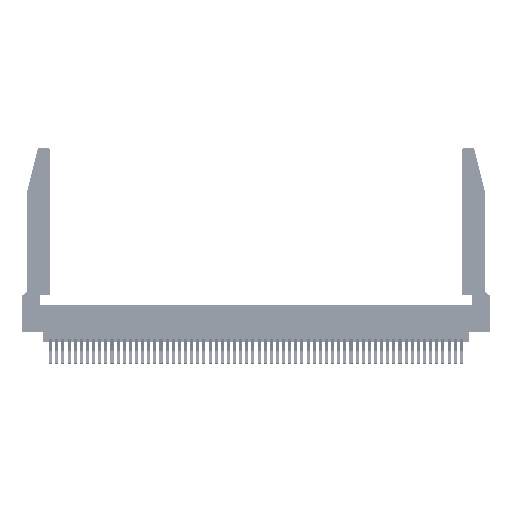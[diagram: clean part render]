
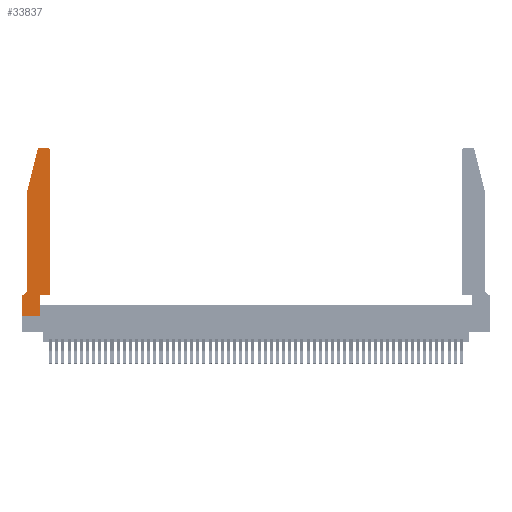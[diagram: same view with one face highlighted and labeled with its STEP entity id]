
A CAD part, top view. The second image highlights one B-rep face of the part: STEP entity #33837.
In plain terms, the highlighted planar face has unit normal (0, 0, 1).
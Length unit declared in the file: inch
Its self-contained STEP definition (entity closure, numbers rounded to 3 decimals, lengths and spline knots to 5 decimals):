
#17 = CARTESIAN_POINT ( 'NONE',  ( 0.2865, 0., 0.37 ) ) ;
#1931 = LINE ( 'NONE', #52127, #19778 ) ;
#2562 = VERTEX_POINT ( 'NONE', #24021 ) ;
#3129 = CARTESIAN_POINT ( 'NONE',  ( 0.4205, 2.75, 0.37 ) ) ;
#3317 = EDGE_CURVE ( 'NONE', #7591, #2562, #39348, .T. ) ;
#3468 = CARTESIAN_POINT ( 'NONE',  ( 0.4205, 2.72, 0.37 ) ) ;
#4200 = ORIENTED_EDGE ( 'NONE', *, *, #9746, .T. ) ;
#6083 = DIRECTION ( 'NONE',  ( 0., 1., 0. ) ) ;
#6955 = CARTESIAN_POINT ( 'NONE',  ( 0.2865, 0.35, 0.37 ) ) ;
#7202 = CIRCLE ( 'NONE', #25815, 0.03 ) ;
#7223 = AXIS2_PLACEMENT_3D ( 'NONE', #47999, #27829, #48746 ) ;
#7579 = EDGE_CURVE ( 'NONE', #15162, #51582, #19291, .T. ) ;
#7591 = VERTEX_POINT ( 'NONE', #15389 ) ;
#7745 = DIRECTION ( 'NONE',  ( 0., 0., 1. ) ) ;
#7972 = EDGE_CURVE ( 'NONE', #21771, #21928, #25898, .T. ) ;
#9334 = DIRECTION ( 'NONE',  ( -1., 0., 0. ) ) ;
#9746 = EDGE_CURVE ( 'NONE', #21928, #7591, #7202, .T. ) ;
#13194 = EDGE_CURVE ( 'NONE', #38398, #21771, #14257, .T. ) ;
#13204 = EDGE_CURVE ( 'NONE', #25595, #15162, #15594, .T. ) ;
#13573 = VERTEX_POINT ( 'NONE', #6955 ) ;
#14257 = CIRCLE ( 'NONE', #15981, 0.03 ) ;
#14456 = VERTEX_POINT ( 'NONE', #46178 ) ;
#15027 = CARTESIAN_POINT ( 'NONE',  ( 0., 0., 0.37 ) ) ;
#15162 = VERTEX_POINT ( 'NONE', #33357 ) ;
#15389 = CARTESIAN_POINT ( 'NONE',  ( 0.25487, 2.72718, 0.37 ) ) ;
#15594 = LINE ( 'NONE', #50302, #30167 ) ;
#15723 = ORIENTED_EDGE ( 'NONE', *, *, #7579, .T. ) ;
#15868 = ORIENTED_EDGE ( 'NONE', *, *, #22685, .T. ) ;
#15981 = AXIS2_PLACEMENT_3D ( 'NONE', #3468, #7745, #45841 ) ;
#16639 = EDGE_CURVE ( 'NONE', #51582, #37300, #1931, .T. ) ;
#17595 = EDGE_LOOP ( 'NONE', ( #52752, #4200, #49155, #15868, #50576, #19796, #15723, #22686, #35357, #24767, #21542, #46918 ) ) ;
#17770 = CARTESIAN_POINT ( 'NONE',  ( 0., 0., 0.37 ) ) ;
#18060 = LINE ( 'NONE', #51191, #53843 ) ;
#18257 = DIRECTION ( 'NONE',  ( -1., 0., 0. ) ) ;
#18615 = CARTESIAN_POINT ( 'NONE',  ( 0.0055, 0.42, 0.37 ) ) ;
#19123 = DIRECTION ( 'NONE',  ( 1., 0., 0. ) ) ;
#19291 = LINE ( 'NONE', #15027, #24624 ) ;
#19778 = VECTOR ( 'NONE', #19123, 39.37008 ) ;
#19796 = ORIENTED_EDGE ( 'NONE', *, *, #13204, .T. ) ;
#19903 = LINE ( 'NONE', #42523, #31259 ) ;
#20831 = VECTOR ( 'NONE', #24140, 39.37008 ) ;
#21542 = ORIENTED_EDGE ( 'NONE', *, *, #47731, .T. ) ;
#21729 = CARTESIAN_POINT ( 'NONE',  ( 0.2605, 2.75, 0.37 ) ) ;
#21771 = VERTEX_POINT ( 'NONE', #3129 ) ;
#21928 = VERTEX_POINT ( 'NONE', #42690 ) ;
#22438 = PLANE ( 'NONE',  #7223 ) ;
#22685 = EDGE_CURVE ( 'NONE', #2562, #24646, #18060, .T. ) ;
#22686 = ORIENTED_EDGE ( 'NONE', *, *, #16639, .T. ) ;
#24021 = CARTESIAN_POINT ( 'NONE',  ( 0.0755, 2., 0.37 ) ) ;
#24140 = DIRECTION ( 'NONE',  ( -0.239, -0.971, 0. ) ) ;
#24413 = CIRCLE ( 'NONE', #53506, 0.07 ) ;
#24624 = VECTOR ( 'NONE', #27620, 39.37008 ) ;
#24646 = VERTEX_POINT ( 'NONE', #38263 ) ;
#24767 = ORIENTED_EDGE ( 'NONE', *, *, #36167, .T. ) ;
#24779 = DIRECTION ( 'NONE',  ( -1., 0., 0. ) ) ;
#25095 = CARTESIAN_POINT ( 'NONE',  ( 0.284, 2.72, 0.37 ) ) ;
#25595 = VERTEX_POINT ( 'NONE', #31531 ) ;
#25815 = AXIS2_PLACEMENT_3D ( 'NONE', #25095, #29510, #33581 ) ;
#25898 = LINE ( 'NONE', #21729, #31195 ) ;
#27004 = VECTOR ( 'NONE', #6083, 39.37008 ) ;
#27512 = DIRECTION ( 'NONE',  ( 0., 0., -1. ) ) ;
#27526 = CARTESIAN_POINT ( 'NONE',  ( 0.4505, 2.72, 0.37 ) ) ;
#27620 = DIRECTION ( 'NONE',  ( 0., -1., 0. ) ) ;
#27829 = DIRECTION ( 'NONE',  ( 0., 0., 1. ) ) ;
#29510 = DIRECTION ( 'NONE',  ( 0., 0., 1. ) ) ;
#29719 = LINE ( 'NONE', #50682, #38977 ) ;
#30167 = VECTOR ( 'NONE', #24779, 39.37008 ) ;
#31169 = DIRECTION ( 'NONE',  ( 0., -1., 0. ) ) ;
#31195 = VECTOR ( 'NONE', #9334, 39.37008 ) ;
#31259 = VECTOR ( 'NONE', #42897, 39.37008 ) ;
#31531 = CARTESIAN_POINT ( 'NONE',  ( 0.0055, 0.35, 0.37 ) ) ;
#33357 = CARTESIAN_POINT ( 'NONE',  ( 0., 0.35, 0.37 ) ) ;
#33462 = DIRECTION ( 'NONE',  ( 1., 0., 0. ) ) ;
#33581 = DIRECTION ( 'NONE',  ( 1., 0., 0. ) ) ;
#33837 = ADVANCED_FACE ( 'NONE', ( #44560 ), #22438, .T. ) ;
#35357 = ORIENTED_EDGE ( 'NONE', *, *, #40311, .T. ) ;
#36167 = EDGE_CURVE ( 'NONE', #13573, #14456, #29719, .T. ) ;
#36404 = EDGE_CURVE ( 'NONE', #24646, #25595, #24413, .T. ) ;
#36699 = CARTESIAN_POINT ( 'NONE',  ( 0.0755, 2., 0.37 ) ) ;
#37300 = VERTEX_POINT ( 'NONE', #17 ) ;
#38263 = CARTESIAN_POINT ( 'NONE',  ( 0.0755, 0.42, 0.37 ) ) ;
#38398 = VERTEX_POINT ( 'NONE', #27526 ) ;
#38977 = VECTOR ( 'NONE', #33462, 39.37008 ) ;
#39348 = LINE ( 'NONE', #36699, #20831 ) ;
#40311 = EDGE_CURVE ( 'NONE', #37300, #13573, #19903, .T. ) ;
#42523 = CARTESIAN_POINT ( 'NONE',  ( 0.2865, 0.35, 0.37 ) ) ;
#42690 = CARTESIAN_POINT ( 'NONE',  ( 0.284, 2.75, 0.37 ) ) ;
#42897 = DIRECTION ( 'NONE',  ( 0., 1., 0. ) ) ;
#44560 = FACE_OUTER_BOUND ( 'NONE', #17595, .T. ) ;
#45841 = DIRECTION ( 'NONE',  ( 1., 0., 0. ) ) ;
#46178 = CARTESIAN_POINT ( 'NONE',  ( 0.4505, 0.35, 0.37 ) ) ;
#46918 = ORIENTED_EDGE ( 'NONE', *, *, #13194, .T. ) ;
#47616 = CARTESIAN_POINT ( 'NONE',  ( 0.4505, 0.35, 0.37 ) ) ;
#47731 = EDGE_CURVE ( 'NONE', #14456, #38398, #48185, .T. ) ;
#47999 = CARTESIAN_POINT ( 'NONE',  ( 0., 0.35, 0.37 ) ) ;
#48185 = LINE ( 'NONE', #47616, #27004 ) ;
#48746 = DIRECTION ( 'NONE',  ( 1., 0., 0. ) ) ;
#49155 = ORIENTED_EDGE ( 'NONE', *, *, #3317, .T. ) ;
#50302 = CARTESIAN_POINT ( 'NONE',  ( 0.0755, 0.35, 0.37 ) ) ;
#50576 = ORIENTED_EDGE ( 'NONE', *, *, #36404, .T. ) ;
#50682 = CARTESIAN_POINT ( 'NONE',  ( 0.4505, 0.35, 0.37 ) ) ;
#51191 = CARTESIAN_POINT ( 'NONE',  ( 0.0755, 2., 0.37 ) ) ;
#51582 = VERTEX_POINT ( 'NONE', #17770 ) ;
#52127 = CARTESIAN_POINT ( 'NONE',  ( 0., 0., 0.37 ) ) ;
#52752 = ORIENTED_EDGE ( 'NONE', *, *, #7972, .T. ) ;
#53506 = AXIS2_PLACEMENT_3D ( 'NONE', #18615, #27512, #18257 ) ;
#53843 = VECTOR ( 'NONE', #31169, 39.37008 ) ;
